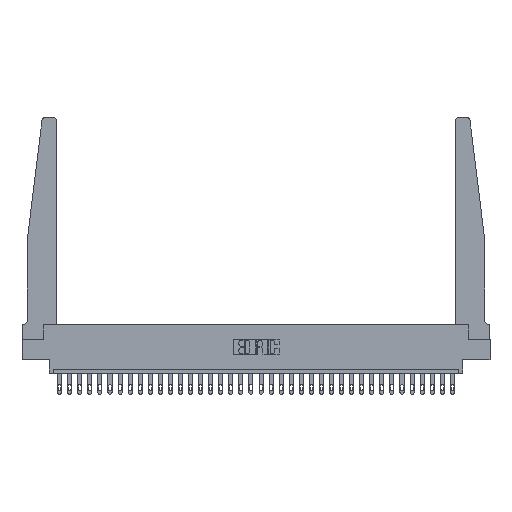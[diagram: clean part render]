
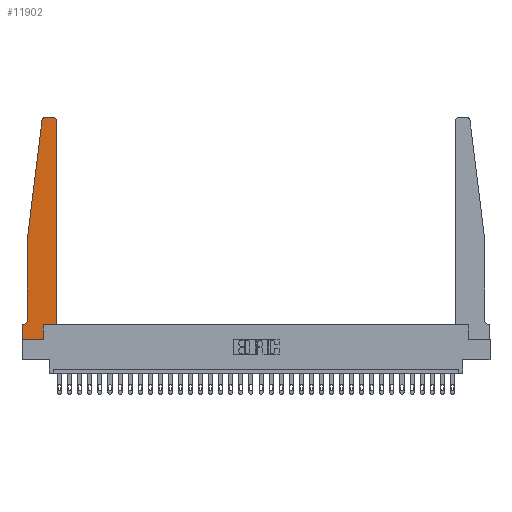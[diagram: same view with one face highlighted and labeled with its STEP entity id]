
A CAD part, top view. The second image highlights one B-rep face of the part: STEP entity #11902.
In plain terms, the highlighted planar face has unit normal (0, 0, 1).
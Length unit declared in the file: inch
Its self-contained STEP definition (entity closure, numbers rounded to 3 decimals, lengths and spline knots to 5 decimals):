
#397 = VERTEX_POINT ( 'NONE', #1815 ) ;
#821 = DIRECTION ( 'NONE',  ( 0., 1., 0. ) ) ;
#876 = CARTESIAN_POINT ( 'NONE',  ( 0.065, 0.1875, 0.37 ) ) ;
#1579 = CIRCLE ( 'NONE', #30035, 0.05 ) ;
#1741 = VECTOR ( 'NONE', #3613, 39.37008 ) ;
#1815 = CARTESIAN_POINT ( 'NONE',  ( 0.425, 2.72, 0.37 ) ) ;
#1997 = EDGE_CURVE ( 'NONE', #8911, #19037, #21885, .T. ) ;
#2199 = CIRCLE ( 'NONE', #20323, 0.03 ) ;
#2792 = ORIENTED_EDGE ( 'NONE', *, *, #25103, .T. ) ;
#3154 = LINE ( 'NONE', #21877, #16508 ) ;
#3215 = CARTESIAN_POINT ( 'NONE',  ( 0.065, 0.2375, 0.37 ) ) ;
#3369 = DIRECTION ( 'NONE',  ( 1., 0., 0. ) ) ;
#3452 = VERTEX_POINT ( 'NONE', #10602 ) ;
#3613 = DIRECTION ( 'NONE',  ( 0., -1., 0. ) ) ;
#3881 = DIRECTION ( 'NONE',  ( 1., 0., 0. ) ) ;
#4944 = CARTESIAN_POINT ( 'NONE',  ( 0.065, 1.25, 0.37 ) ) ;
#5674 = VERTEX_POINT ( 'NONE', #20814 ) ;
#5738 = DIRECTION ( 'NONE',  ( 0., 0., -1. ) ) ;
#5922 = CARTESIAN_POINT ( 'NONE',  ( 0., 0., 0.37 ) ) ;
#6216 = LINE ( 'NONE', #15584, #16226 ) ;
#6510 = ORIENTED_EDGE ( 'NONE', *, *, #30332, .T. ) ;
#7089 = CARTESIAN_POINT ( 'NONE',  ( 0.27653, 2.75, 0.37 ) ) ;
#8656 = ORIENTED_EDGE ( 'NONE', *, *, #25042, .T. ) ;
#8784 = CARTESIAN_POINT ( 'NONE',  ( 0., 0., 0.37 ) ) ;
#8823 = LINE ( 'NONE', #15889, #15546 ) ;
#8911 = VERTEX_POINT ( 'NONE', #12533 ) ;
#9297 = EDGE_CURVE ( 'NONE', #21009, #8911, #1579, .T. ) ;
#9627 = VECTOR ( 'NONE', #3369, 39.37008 ) ;
#10138 = DIRECTION ( 'NONE',  ( -0.122, -0.992, 0. ) ) ;
#10173 = PLANE ( 'NONE',  #25209 ) ;
#10579 = LINE ( 'NONE', #24550, #9627 ) ;
#10602 = CARTESIAN_POINT ( 'NONE',  ( 0.395, 2.75, 0.37 ) ) ;
#11876 = EDGE_CURVE ( 'NONE', #21157, #397, #12485, .T. ) ;
#11902 = ADVANCED_FACE ( 'NONE', ( #19381 ), #10173, .T. ) ;
#12037 = EDGE_CURVE ( 'NONE', #397, #3452, #2199, .T. ) ;
#12274 = CARTESIAN_POINT ( 'NONE',  ( 0., 0., 0.37 ) ) ;
#12302 = LINE ( 'NONE', #4944, #27002 ) ;
#12485 = LINE ( 'NONE', #28308, #17365 ) ;
#12533 = CARTESIAN_POINT ( 'NONE',  ( 0.015, 0.1875, 0.37 ) ) ;
#12649 = CARTESIAN_POINT ( 'NONE',  ( 0.24675, 2.72367, 0.37 ) ) ;
#12771 = ORIENTED_EDGE ( 'NONE', *, *, #1997, .T. ) ;
#14747 = EDGE_CURVE ( 'NONE', #19037, #18441, #26805, .T. ) ;
#14923 = DIRECTION ( 'NONE',  ( 1., 0., 0. ) ) ;
#15058 = CIRCLE ( 'NONE', #25850, 0.03 ) ;
#15370 = ORIENTED_EDGE ( 'NONE', *, *, #11876, .T. ) ;
#15546 = VECTOR ( 'NONE', #17738, 39.37008 ) ;
#15584 = CARTESIAN_POINT ( 'NONE',  ( 0.25, 2.75, 0.37 ) ) ;
#15889 = CARTESIAN_POINT ( 'NONE',  ( 0.065, 1.25, 0.37 ) ) ;
#15890 = DIRECTION ( 'NONE',  ( -1., 0., 0. ) ) ;
#16011 = ORIENTED_EDGE ( 'NONE', *, *, #23662, .T. ) ;
#16226 = VECTOR ( 'NONE', #15890, 39.37008 ) ;
#16508 = VECTOR ( 'NONE', #28957, 39.37008 ) ;
#16670 = DIRECTION ( 'NONE',  ( 1., 0., 0. ) ) ;
#17365 = VECTOR ( 'NONE', #821, 39.37008 ) ;
#17550 = CARTESIAN_POINT ( 'NONE',  ( 0.395, 2.72, 0.37 ) ) ;
#17562 = DIRECTION ( 'NONE',  ( -1., 0., 0. ) ) ;
#17738 = DIRECTION ( 'NONE',  ( 0., -1., 0. ) ) ;
#18027 = ORIENTED_EDGE ( 'NONE', *, *, #29812, .T. ) ;
#18400 = VECTOR ( 'NONE', #24194, 39.37008 ) ;
#18441 = VERTEX_POINT ( 'NONE', #12274 ) ;
#19037 = VERTEX_POINT ( 'NONE', #22466 ) ;
#19381 = FACE_OUTER_BOUND ( 'NONE', #28089, .T. ) ;
#20323 = AXIS2_PLACEMENT_3D ( 'NONE', #17550, #29069, #14923 ) ;
#20814 = CARTESIAN_POINT ( 'NONE',  ( 0.2605, 0.18, 0.37 ) ) ;
#21009 = VERTEX_POINT ( 'NONE', #3215 ) ;
#21157 = VERTEX_POINT ( 'NONE', #24697 ) ;
#21226 = ORIENTED_EDGE ( 'NONE', *, *, #14747, .T. ) ;
#21422 = CARTESIAN_POINT ( 'NONE',  ( 0.27653, 2.72, 0.37 ) ) ;
#21870 = DIRECTION ( 'NONE',  ( 0., 0., 1. ) ) ;
#21877 = CARTESIAN_POINT ( 'NONE',  ( 0.2605, 0.18, 0.37 ) ) ;
#21885 = LINE ( 'NONE', #876, #18400 ) ;
#22214 = ORIENTED_EDGE ( 'NONE', *, *, #12037, .T. ) ;
#22463 = ORIENTED_EDGE ( 'NONE', *, *, #29278, .T. ) ;
#22466 = CARTESIAN_POINT ( 'NONE',  ( 0., 0.1875, 0.37 ) ) ;
#22994 = EDGE_CURVE ( 'NONE', #5674, #21157, #10579, .T. ) ;
#23364 = ORIENTED_EDGE ( 'NONE', *, *, #9297, .T. ) ;
#23527 = DIRECTION ( 'NONE',  ( 1., 0., 0. ) ) ;
#23662 = EDGE_CURVE ( 'NONE', #25717, #26644, #15058, .T. ) ;
#24146 = DIRECTION ( 'NONE',  ( 0., 0., 1. ) ) ;
#24194 = DIRECTION ( 'NONE',  ( -1., 0., 0. ) ) ;
#24273 = VERTEX_POINT ( 'NONE', #29669 ) ;
#24550 = CARTESIAN_POINT ( 'NONE',  ( 0.425, 0.18, 0.37 ) ) ;
#24697 = CARTESIAN_POINT ( 'NONE',  ( 0.425, 0.18, 0.37 ) ) ;
#24907 = LINE ( 'NONE', #8784, #28021 ) ;
#25042 = EDGE_CURVE ( 'NONE', #24273, #5674, #3154, .T. ) ;
#25103 = EDGE_CURVE ( 'NONE', #26252, #21009, #8823, .T. ) ;
#25209 = AXIS2_PLACEMENT_3D ( 'NONE', #26147, #24146, #23527 ) ;
#25717 = VERTEX_POINT ( 'NONE', #7089 ) ;
#25850 = AXIS2_PLACEMENT_3D ( 'NONE', #21422, #21870, #16670 ) ;
#26147 = CARTESIAN_POINT ( 'NONE',  ( 0., 0.1875, 0.37 ) ) ;
#26252 = VERTEX_POINT ( 'NONE', #28544 ) ;
#26644 = VERTEX_POINT ( 'NONE', #12649 ) ;
#26767 = CARTESIAN_POINT ( 'NONE',  ( 0.015, 0.2375, 0.37 ) ) ;
#26805 = LINE ( 'NONE', #5922, #1741 ) ;
#27002 = VECTOR ( 'NONE', #10138, 39.37008 ) ;
#27905 = ORIENTED_EDGE ( 'NONE', *, *, #22994, .T. ) ;
#28021 = VECTOR ( 'NONE', #3881, 39.37008 ) ;
#28089 = EDGE_LOOP ( 'NONE', ( #18027, #16011, #22463, #2792, #23364, #12771, #21226, #6510, #8656, #27905, #15370, #22214 ) ) ;
#28308 = CARTESIAN_POINT ( 'NONE',  ( 0.425, 0.18, 0.37 ) ) ;
#28544 = CARTESIAN_POINT ( 'NONE',  ( 0.065, 1.25, 0.37 ) ) ;
#28957 = DIRECTION ( 'NONE',  ( 0., 1., 0. ) ) ;
#29069 = DIRECTION ( 'NONE',  ( 0., 0., 1. ) ) ;
#29278 = EDGE_CURVE ( 'NONE', #26644, #26252, #12302, .T. ) ;
#29669 = CARTESIAN_POINT ( 'NONE',  ( 0.2605, 0., 0.37 ) ) ;
#29812 = EDGE_CURVE ( 'NONE', #3452, #25717, #6216, .T. ) ;
#30035 = AXIS2_PLACEMENT_3D ( 'NONE', #26767, #5738, #17562 ) ;
#30332 = EDGE_CURVE ( 'NONE', #18441, #24273, #24907, .T. ) ;
